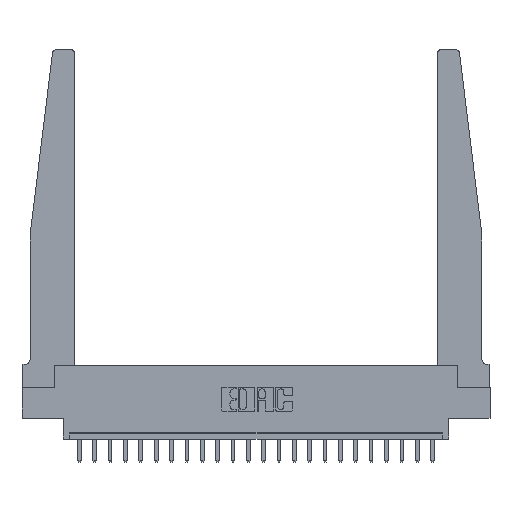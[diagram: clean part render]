
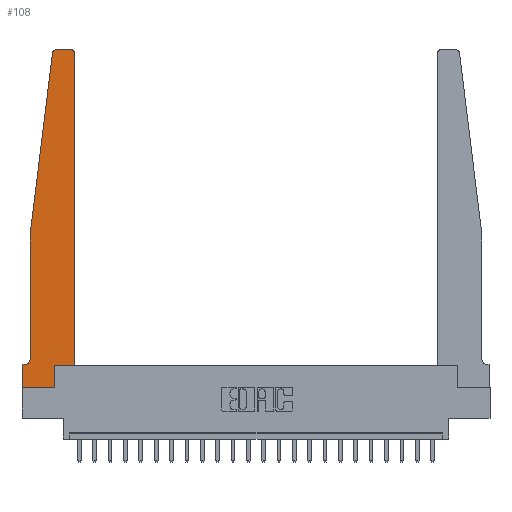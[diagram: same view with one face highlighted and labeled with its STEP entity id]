
A CAD part, top view. The second image highlights one B-rep face of the part: STEP entity #108.
In plain terms, the highlighted planar face has unit normal (0, 0, 1).
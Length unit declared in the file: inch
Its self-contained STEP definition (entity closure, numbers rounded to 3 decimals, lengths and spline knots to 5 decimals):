
#46 = EDGE_CURVE ( 'NONE', #11918, #14090, #6768, .T. ) ;
#108 = ADVANCED_FACE ( 'NONE', ( #20797 ), #14438, .T. ) ;
#393 = CARTESIAN_POINT ( 'NONE',  ( 0., 0., 0.37 ) ) ;
#672 = ORIENTED_EDGE ( 'NONE', *, *, #18381, .T. ) ;
#1091 = LINE ( 'NONE', #8420, #3254 ) ;
#1142 = CARTESIAN_POINT ( 'NONE',  ( 0.065, 0.1875, 0.37 ) ) ;
#1400 = EDGE_CURVE ( 'NONE', #17181, #8283, #13234, .T. ) ;
#1471 = CARTESIAN_POINT ( 'NONE',  ( 0.065, 1.25, 0.37 ) ) ;
#1788 = AXIS2_PLACEMENT_3D ( 'NONE', #16388, #5890, #14510 ) ;
#2452 = ORIENTED_EDGE ( 'NONE', *, *, #2955, .T. ) ;
#2955 = EDGE_CURVE ( 'NONE', #7458, #17181, #11505, .T. ) ;
#3254 = VECTOR ( 'NONE', #11802, 39.37008 ) ;
#3346 = ORIENTED_EDGE ( 'NONE', *, *, #5673, .T. ) ;
#3347 = CARTESIAN_POINT ( 'NONE',  ( 0.065, 1.25, 0.37 ) ) ;
#3572 = CIRCLE ( 'NONE', #13695, 0.03 ) ;
#3618 = CARTESIAN_POINT ( 'NONE',  ( 0.395, 2.75, 0.37 ) ) ;
#4258 = DIRECTION ( 'NONE',  ( 0., 0., 1. ) ) ;
#4370 = ORIENTED_EDGE ( 'NONE', *, *, #1400, .T. ) ;
#4487 = LINE ( 'NONE', #1142, #21439 ) ;
#4795 = CARTESIAN_POINT ( 'NONE',  ( 0.2605, 0., 0.37 ) ) ;
#4995 = EDGE_LOOP ( 'NONE', ( #9006, #10227, #672, #7837, #15198, #3346, #20629, #2452, #4370, #16253, #9882, #13404 ) ) ;
#5332 = CARTESIAN_POINT ( 'NONE',  ( 0., 0.1875, 0.37 ) ) ;
#5673 = EDGE_CURVE ( 'NONE', #14090, #9051, #4487, .T. ) ;
#5890 = DIRECTION ( 'NONE',  ( 0., 0., -1. ) ) ;
#5929 = VERTEX_POINT ( 'NONE', #8958 ) ;
#5933 = DIRECTION ( 'NONE',  ( 0., 0., 1. ) ) ;
#6467 = DIRECTION ( 'NONE',  ( 1., 0., 0. ) ) ;
#6768 = CIRCLE ( 'NONE', #1788, 0.05 ) ;
#6960 = DIRECTION ( 'NONE',  ( 0., 1., 0. ) ) ;
#7042 = DIRECTION ( 'NONE',  ( -0.122, -0.992, 0. ) ) ;
#7276 = VECTOR ( 'NONE', #7042, 39.37008 ) ;
#7458 = VERTEX_POINT ( 'NONE', #393 ) ;
#7837 = ORIENTED_EDGE ( 'NONE', *, *, #8946, .T. ) ;
#7992 = AXIS2_PLACEMENT_3D ( 'NONE', #16159, #12954, #14366 ) ;
#8096 = CARTESIAN_POINT ( 'NONE',  ( 0.25, 2.75, 0.37 ) ) ;
#8109 = VECTOR ( 'NONE', #15452, 39.37008 ) ;
#8283 = VERTEX_POINT ( 'NONE', #11864 ) ;
#8420 = CARTESIAN_POINT ( 'NONE',  ( 0.425, 0.18, 0.37 ) ) ;
#8946 = EDGE_CURVE ( 'NONE', #12864, #11918, #14375, .T. ) ;
#8958 = CARTESIAN_POINT ( 'NONE',  ( 0.27653, 2.75, 0.37 ) ) ;
#9006 = ORIENTED_EDGE ( 'NONE', *, *, #18346, .T. ) ;
#9051 = VERTEX_POINT ( 'NONE', #5332 ) ;
#9679 = VECTOR ( 'NONE', #16117, 39.37008 ) ;
#9828 = LINE ( 'NONE', #18623, #16593 ) ;
#9882 = ORIENTED_EDGE ( 'NONE', *, *, #17923, .T. ) ;
#9922 = EDGE_CURVE ( 'NONE', #12088, #15563, #11448, .T. ) ;
#10197 = VECTOR ( 'NONE', #6960, 39.37008 ) ;
#10227 = ORIENTED_EDGE ( 'NONE', *, *, #10570, .T. ) ;
#10570 = EDGE_CURVE ( 'NONE', #5929, #12485, #3572, .T. ) ;
#11448 = CIRCLE ( 'NONE', #21141, 0.03 ) ;
#11505 = LINE ( 'NONE', #18136, #19041 ) ;
#11802 = DIRECTION ( 'NONE',  ( 0., 1., 0. ) ) ;
#11864 = CARTESIAN_POINT ( 'NONE',  ( 0.2605, 0.18, 0.37 ) ) ;
#11918 = VERTEX_POINT ( 'NONE', #17472 ) ;
#12049 = CARTESIAN_POINT ( 'NONE',  ( 0.2605, 0.18, 0.37 ) ) ;
#12088 = VERTEX_POINT ( 'NONE', #16508 ) ;
#12133 = CARTESIAN_POINT ( 'NONE',  ( 0.425, 0.18, 0.37 ) ) ;
#12442 = CARTESIAN_POINT ( 'NONE',  ( 0.065, 1.25, 0.37 ) ) ;
#12485 = VERTEX_POINT ( 'NONE', #14245 ) ;
#12503 = EDGE_CURVE ( 'NONE', #9051, #7458, #13785, .T. ) ;
#12864 = VERTEX_POINT ( 'NONE', #12442 ) ;
#12903 = CARTESIAN_POINT ( 'NONE',  ( 0.395, 2.72, 0.37 ) ) ;
#12954 = DIRECTION ( 'NONE',  ( 0., 0., 1. ) ) ;
#13046 = DIRECTION ( 'NONE',  ( 1., 0., 0. ) ) ;
#13234 = LINE ( 'NONE', #12049, #10197 ) ;
#13404 = ORIENTED_EDGE ( 'NONE', *, *, #9922, .T. ) ;
#13436 = DIRECTION ( 'NONE',  ( -1., 0., 0. ) ) ;
#13695 = AXIS2_PLACEMENT_3D ( 'NONE', #14624, #5933, #17998 ) ;
#13785 = LINE ( 'NONE', #19481, #9679 ) ;
#14090 = VERTEX_POINT ( 'NONE', #20605 ) ;
#14245 = CARTESIAN_POINT ( 'NONE',  ( 0.24675, 2.72367, 0.37 ) ) ;
#14366 = DIRECTION ( 'NONE',  ( 1., 0., 0. ) ) ;
#14369 = VERTEX_POINT ( 'NONE', #12133 ) ;
#14375 = LINE ( 'NONE', #1471, #8109 ) ;
#14438 = PLANE ( 'NONE',  #7992 ) ;
#14510 = DIRECTION ( 'NONE',  ( -1., 0., 0. ) ) ;
#14624 = CARTESIAN_POINT ( 'NONE',  ( 0.27653, 2.72, 0.37 ) ) ;
#15198 = ORIENTED_EDGE ( 'NONE', *, *, #46, .T. ) ;
#15452 = DIRECTION ( 'NONE',  ( 0., -1., 0. ) ) ;
#15563 = VERTEX_POINT ( 'NONE', #3618 ) ;
#16117 = DIRECTION ( 'NONE',  ( 0., -1., 0. ) ) ;
#16159 = CARTESIAN_POINT ( 'NONE',  ( 0., 0.1875, 0.37 ) ) ;
#16253 = ORIENTED_EDGE ( 'NONE', *, *, #21686, .T. ) ;
#16388 = CARTESIAN_POINT ( 'NONE',  ( 0.015, 0.2375, 0.37 ) ) ;
#16508 = CARTESIAN_POINT ( 'NONE',  ( 0.425, 2.72, 0.37 ) ) ;
#16593 = VECTOR ( 'NONE', #6467, 39.37008 ) ;
#16715 = LINE ( 'NONE', #3347, #7276 ) ;
#17181 = VERTEX_POINT ( 'NONE', #4795 ) ;
#17256 = LINE ( 'NONE', #8096, #18880 ) ;
#17472 = CARTESIAN_POINT ( 'NONE',  ( 0.065, 0.2375, 0.37 ) ) ;
#17923 = EDGE_CURVE ( 'NONE', #14369, #12088, #1091, .T. ) ;
#17998 = DIRECTION ( 'NONE',  ( 1., 0., 0. ) ) ;
#18136 = CARTESIAN_POINT ( 'NONE',  ( 0., 0., 0.37 ) ) ;
#18346 = EDGE_CURVE ( 'NONE', #15563, #5929, #17256, .T. ) ;
#18381 = EDGE_CURVE ( 'NONE', #12485, #12864, #16715, .T. ) ;
#18623 = CARTESIAN_POINT ( 'NONE',  ( 0.425, 0.18, 0.37 ) ) ;
#18880 = VECTOR ( 'NONE', #13436, 39.37008 ) ;
#19041 = VECTOR ( 'NONE', #19856, 39.37008 ) ;
#19481 = CARTESIAN_POINT ( 'NONE',  ( 0., 0., 0.37 ) ) ;
#19856 = DIRECTION ( 'NONE',  ( 1., 0., 0. ) ) ;
#20067 = DIRECTION ( 'NONE',  ( -1., 0., 0. ) ) ;
#20605 = CARTESIAN_POINT ( 'NONE',  ( 0.015, 0.1875, 0.37 ) ) ;
#20629 = ORIENTED_EDGE ( 'NONE', *, *, #12503, .T. ) ;
#20797 = FACE_OUTER_BOUND ( 'NONE', #4995, .T. ) ;
#21141 = AXIS2_PLACEMENT_3D ( 'NONE', #12903, #4258, #13046 ) ;
#21439 = VECTOR ( 'NONE', #20067, 39.37008 ) ;
#21686 = EDGE_CURVE ( 'NONE', #8283, #14369, #9828, .T. ) ;
